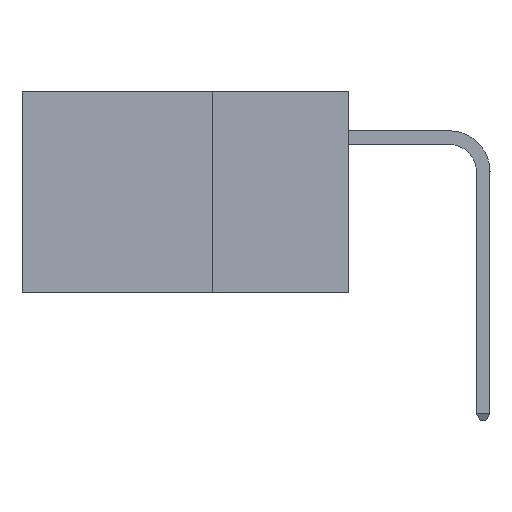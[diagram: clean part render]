
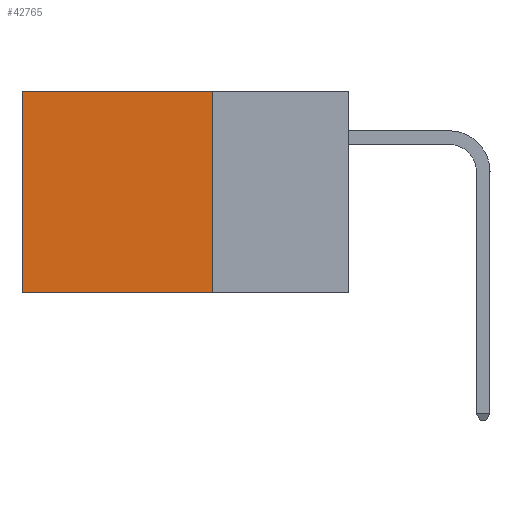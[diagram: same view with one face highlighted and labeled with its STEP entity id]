
A CAD part, left-side view. The second image highlights one B-rep face of the part: STEP entity #42765.
In plain terms, the highlighted planar face has unit normal (-1, 0, 0).
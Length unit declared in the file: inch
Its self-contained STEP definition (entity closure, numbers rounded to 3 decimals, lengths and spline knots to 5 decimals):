
#1422 = VERTEX_POINT ( 'NONE', #15885 ) ;
#2212 = CARTESIAN_POINT ( 'NONE',  ( 0.2875, 0.25, -0.37 ) ) ;
#5951 = CARTESIAN_POINT ( 'NONE',  ( 0.2875, 0.6, 0. ) ) ;
#7065 = DIRECTION ( 'NONE',  ( 0., 1., 0. ) ) ;
#7739 = VECTOR ( 'NONE', #7065, 39.37008 ) ;
#8138 = VERTEX_POINT ( 'NONE', #5951 ) ;
#10775 = CARTESIAN_POINT ( 'NONE',  ( 0.2875, 0.25, 0. ) ) ;
#12162 = LINE ( 'NONE', #19526, #48453 ) ;
#12388 = EDGE_CURVE ( 'NONE', #44135, #44851, #12162, .T. ) ;
#13432 = CARTESIAN_POINT ( 'NONE',  ( 0.2875, 0.25, 0. ) ) ;
#13599 = DIRECTION ( 'NONE',  ( 0., 0., -1. ) ) ;
#15763 = ORIENTED_EDGE ( 'NONE', *, *, #31501, .T. ) ;
#15885 = CARTESIAN_POINT ( 'NONE',  ( 0.2875, 0.6, -0.37 ) ) ;
#16945 = DIRECTION ( 'NONE',  ( 0., 0., -1. ) ) ;
#19526 = CARTESIAN_POINT ( 'NONE',  ( 0.2875, 0.25, 0. ) ) ;
#25921 = ORIENTED_EDGE ( 'NONE', *, *, #12388, .F. ) ;
#26094 = VECTOR ( 'NONE', #16945, 39.37008 ) ;
#26416 = DIRECTION ( 'NONE',  ( 0., 1., 0. ) ) ;
#26611 = ORIENTED_EDGE ( 'NONE', *, *, #33734, .F. ) ;
#27857 = AXIS2_PLACEMENT_3D ( 'NONE', #13432, #40458, #13599 ) ;
#29212 = CARTESIAN_POINT ( 'NONE',  ( 0.2875, 0.6, 0. ) ) ;
#30061 = EDGE_CURVE ( 'NONE', #8138, #1422, #31496, .T. ) ;
#30459 = FACE_OUTER_BOUND ( 'NONE', #30937, .T. ) ;
#30937 = EDGE_LOOP ( 'NONE', ( #33942, #26611, #25921, #15763 ) ) ;
#31496 = LINE ( 'NONE', #29212, #26094 ) ;
#31501 = EDGE_CURVE ( 'NONE', #44135, #8138, #42167, .T. ) ;
#33734 = EDGE_CURVE ( 'NONE', #44851, #1422, #35940, .T. ) ;
#33942 = ORIENTED_EDGE ( 'NONE', *, *, #30061, .T. ) ;
#35826 = CARTESIAN_POINT ( 'NONE',  ( 0.2875, 0.25, -0.37 ) ) ;
#35940 = LINE ( 'NONE', #2212, #47403 ) ;
#40458 = DIRECTION ( 'NONE',  ( 1., 0., 0. ) ) ;
#40624 = PLANE ( 'NONE',  #27857 ) ;
#42167 = LINE ( 'NONE', #10775, #7739 ) ;
#42520 = CARTESIAN_POINT ( 'NONE',  ( 0.2875, 0.25, 0. ) ) ;
#42765 = ADVANCED_FACE ( 'NONE', ( #30459 ), #40624, .F. ) ;
#44135 = VERTEX_POINT ( 'NONE', #42520 ) ;
#44851 = VERTEX_POINT ( 'NONE', #35826 ) ;
#46875 = DIRECTION ( 'NONE',  ( 0., 0., -1. ) ) ;
#47403 = VECTOR ( 'NONE', #26416, 39.37008 ) ;
#48453 = VECTOR ( 'NONE', #46875, 39.37008 ) ;
